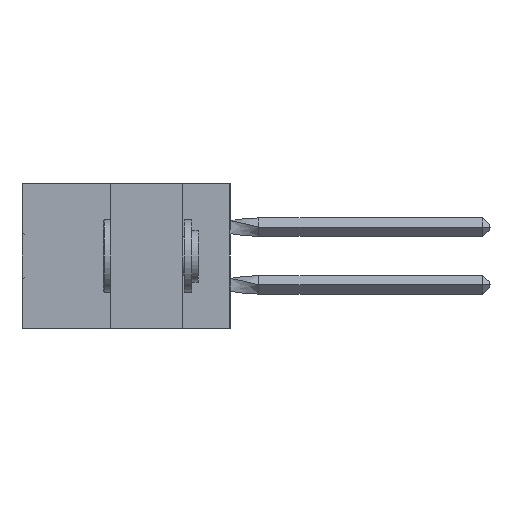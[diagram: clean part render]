
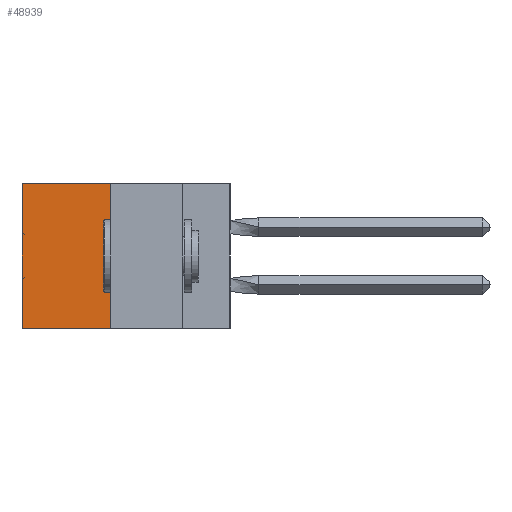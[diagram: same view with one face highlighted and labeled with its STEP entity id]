
A CAD part, left-side view. The second image highlights one B-rep face of the part: STEP entity #48939.
In plain terms, the highlighted planar face has unit normal (-1, 0, 0).
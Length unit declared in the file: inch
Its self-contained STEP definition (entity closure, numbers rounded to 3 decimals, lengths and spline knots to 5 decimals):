
#151 = CARTESIAN_POINT ( 'NONE',  ( 0.305, 0.413, 0. ) ) ;
#708 = CARTESIAN_POINT ( 'NONE',  ( 0.305, 0.413, -0.5 ) ) ;
#1053 = CARTESIAN_POINT ( 'NONE',  ( 0.305, 0.413, -0.5 ) ) ;
#1367 = FACE_OUTER_BOUND ( 'NONE', #30813, .T. ) ;
#2786 = ORIENTED_EDGE ( 'NONE', *, *, #50946, .T. ) ;
#3480 = CARTESIAN_POINT ( 'NONE',  ( 0.305, 0.413, 0. ) ) ;
#3602 = DIRECTION ( 'NONE',  ( 0., 1., 0. ) ) ;
#4714 = DIRECTION ( 'NONE',  ( 0., 0., -1. ) ) ;
#4964 = CARTESIAN_POINT ( 'NONE',  ( 0.305, 0.72, -0.5 ) ) ;
#7237 = VERTEX_POINT ( 'NONE', #14486 ) ;
#9688 = DIRECTION ( 'NONE',  ( 0., 0., -1. ) ) ;
#12526 = DIRECTION ( 'NONE',  ( 0., 0., -1. ) ) ;
#13334 = VERTEX_POINT ( 'NONE', #1053 ) ;
#14486 = CARTESIAN_POINT ( 'NONE',  ( 0.305, 0.72, 0. ) ) ;
#14594 = LINE ( 'NONE', #4964, #49232 ) ;
#15644 = ORIENTED_EDGE ( 'NONE', *, *, #22316, .F. ) ;
#15879 = CARTESIAN_POINT ( 'NONE',  ( 0.305, 0.413, -0.5 ) ) ;
#18146 = LINE ( 'NONE', #21413, #28314 ) ;
#21413 = CARTESIAN_POINT ( 'NONE',  ( 0.305, 0.413, -0.5 ) ) ;
#22167 = VECTOR ( 'NONE', #47885, 39.37008 ) ;
#22316 = EDGE_CURVE ( 'NONE', #33498, #13334, #18146, .T. ) ;
#22637 = VERTEX_POINT ( 'NONE', #27749 ) ;
#23835 = ORIENTED_EDGE ( 'NONE', *, *, #36667, .F. ) ;
#27749 = CARTESIAN_POINT ( 'NONE',  ( 0.305, 0.72, -0.5 ) ) ;
#28314 = VECTOR ( 'NONE', #12526, 39.37008 ) ;
#30813 = EDGE_LOOP ( 'NONE', ( #35663, #23835, #15644, #2786 ) ) ;
#33498 = VERTEX_POINT ( 'NONE', #3480 ) ;
#33656 = LINE ( 'NONE', #151, #22167 ) ;
#34945 = LINE ( 'NONE', #15879, #53284 ) ;
#35663 = ORIENTED_EDGE ( 'NONE', *, *, #51513, .T. ) ;
#36546 = AXIS2_PLACEMENT_3D ( 'NONE', #708, #39508, #4714 ) ;
#36667 = EDGE_CURVE ( 'NONE', #13334, #22637, #34945, .T. ) ;
#39508 = DIRECTION ( 'NONE',  ( 1., 0., 0. ) ) ;
#47885 = DIRECTION ( 'NONE',  ( 0., 1., 0. ) ) ;
#47901 = PLANE ( 'NONE',  #36546 ) ;
#48939 = ADVANCED_FACE ( 'NONE', ( #1367 ), #47901, .F. ) ;
#49232 = VECTOR ( 'NONE', #9688, 39.37008 ) ;
#50946 = EDGE_CURVE ( 'NONE', #33498, #7237, #33656, .T. ) ;
#51513 = EDGE_CURVE ( 'NONE', #7237, #22637, #14594, .T. ) ;
#53284 = VECTOR ( 'NONE', #3602, 39.37008 ) ;
